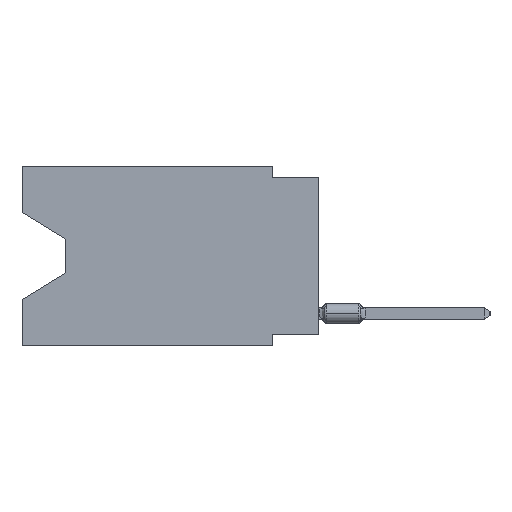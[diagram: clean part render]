
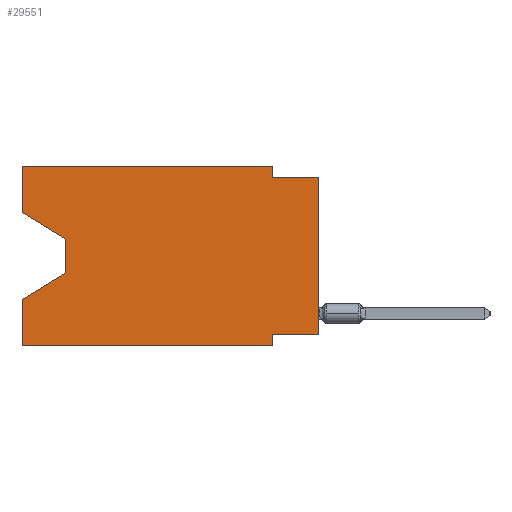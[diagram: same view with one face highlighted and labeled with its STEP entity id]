
A CAD part, left-side view. The second image highlights one B-rep face of the part: STEP entity #29551.
In plain terms, the highlighted planar face has unit normal (-1, 0, 0).
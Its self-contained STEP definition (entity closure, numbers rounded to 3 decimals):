
#448 = LINE ( 'NONE', #6005, #9461 ) ;
#679 = LINE ( 'NONE', #26316, #11996 ) ;
#775 = CARTESIAN_POINT ( 'NONE',  ( 0., 2.54, 0. ) ) ;
#1828 = VECTOR ( 'NONE', #32775, 1000. ) ;
#2061 = VERTEX_POINT ( 'NONE', #11867 ) ;
#2332 = ORIENTED_EDGE ( 'NONE', *, *, #27946, .T. ) ;
#2403 = AXIS2_PLACEMENT_3D ( 'NONE', #29248, #6154, #24351 ) ;
#2508 = CARTESIAN_POINT ( 'NONE',  ( 0., 0., -0.635 ) ) ;
#2751 = EDGE_CURVE ( 'NONE', #22039, #10640, #679, .T. ) ;
#3446 = CARTESIAN_POINT ( 'NONE',  ( 0., 13.97, -5.893 ) ) ;
#3565 = CARTESIAN_POINT ( 'NONE',  ( 0., 2.54, -0.635 ) ) ;
#3770 = LINE ( 'NONE', #4267, #6406 ) ;
#4206 = ORIENTED_EDGE ( 'NONE', *, *, #32711, .F. ) ;
#4267 = CARTESIAN_POINT ( 'NONE',  ( 0., 0., 0. ) ) ;
#4527 = VECTOR ( 'NONE', #31178, 1000. ) ;
#4902 = EDGE_CURVE ( 'NONE', #11299, #10640, #3770, .T. ) ;
#5453 = DIRECTION ( 'NONE',  ( 0., 1., 0. ) ) ;
#5502 = DIRECTION ( 'NONE',  ( 0., -0.855, -0.519 ) ) ;
#5620 = LINE ( 'NONE', #18114, #32018 ) ;
#5708 = DIRECTION ( 'NONE',  ( 0., -1., 0. ) ) ;
#5811 = VERTEX_POINT ( 'NONE', #30617 ) ;
#5850 = CARTESIAN_POINT ( 'NONE',  ( 0., 16.383, -7.36 ) ) ;
#6005 = CARTESIAN_POINT ( 'NONE',  ( 0., 16.383, -2.546 ) ) ;
#6154 = DIRECTION ( 'NONE',  ( 1., 0., 0. ) ) ;
#6406 = VECTOR ( 'NONE', #21792, 1000. ) ;
#7443 = LINE ( 'NONE', #9958, #22364 ) ;
#7466 = EDGE_CURVE ( 'NONE', #18570, #10841, #23406, .T. ) ;
#7983 = EDGE_CURVE ( 'NONE', #12287, #2061, #448, .T. ) ;
#8446 = DIRECTION ( 'NONE',  ( 0., -1., 0. ) ) ;
#8540 = EDGE_CURVE ( 'NONE', #11299, #9713, #5620, .T. ) ;
#8933 = LINE ( 'NONE', #24431, #16962 ) ;
#8987 = VERTEX_POINT ( 'NONE', #775 ) ;
#9274 = VERTEX_POINT ( 'NONE', #27736 ) ;
#9461 = VECTOR ( 'NONE', #5502, 1000. ) ;
#9598 = DIRECTION ( 'NONE',  ( 0., 0., -1. ) ) ;
#9713 = VERTEX_POINT ( 'NONE', #28041 ) ;
#9806 = EDGE_CURVE ( 'NONE', #8987, #22039, #18074, .T. ) ;
#9958 = CARTESIAN_POINT ( 'NONE',  ( 0., 2.54, -9.906 ) ) ;
#10609 = CARTESIAN_POINT ( 'NONE',  ( 0., 16.383, 0. ) ) ;
#10640 = VERTEX_POINT ( 'NONE', #2508 ) ;
#10841 = VERTEX_POINT ( 'NONE', #5850 ) ;
#11116 = ORIENTED_EDGE ( 'NONE', *, *, #14763, .F. ) ;
#11299 = VERTEX_POINT ( 'NONE', #20805 ) ;
#11867 = CARTESIAN_POINT ( 'NONE',  ( 0., 13.97, -4.013 ) ) ;
#11996 = VECTOR ( 'NONE', #8446, 1000. ) ;
#12287 = VERTEX_POINT ( 'NONE', #14750 ) ;
#12697 = CARTESIAN_POINT ( 'NONE',  ( 0., 16.383, -9.906 ) ) ;
#13903 = PLANE ( 'NONE',  #2403 ) ;
#14079 = EDGE_CURVE ( 'NONE', #18570, #9274, #14881, .T. ) ;
#14750 = CARTESIAN_POINT ( 'NONE',  ( 0., 16.383, -2.546 ) ) ;
#14763 = EDGE_CURVE ( 'NONE', #5811, #8987, #23402, .T. ) ;
#14881 = LINE ( 'NONE', #12697, #1828 ) ;
#15157 = ORIENTED_EDGE ( 'NONE', *, *, #31371, .F. ) ;
#15561 = VECTOR ( 'NONE', #16416, 1000. ) ;
#16416 = DIRECTION ( 'NONE',  ( 0., 0.855, -0.519 ) ) ;
#16758 = FACE_OUTER_BOUND ( 'NONE', #26037, .T. ) ;
#16962 = VECTOR ( 'NONE', #32370, 1000. ) ;
#17467 = VECTOR ( 'NONE', #5708, 1000. ) ;
#18067 = ORIENTED_EDGE ( 'NONE', *, *, #8540, .F. ) ;
#18074 = LINE ( 'NONE', #20750, #31815 ) ;
#18114 = CARTESIAN_POINT ( 'NONE',  ( 0., 0., -9.271 ) ) ;
#18570 = VERTEX_POINT ( 'NONE', #31548 ) ;
#19299 = VERTEX_POINT ( 'NONE', #25590 ) ;
#20232 = DIRECTION ( 'NONE',  ( 0., 0., -1. ) ) ;
#20750 = CARTESIAN_POINT ( 'NONE',  ( 0., 2.54, 0. ) ) ;
#20805 = CARTESIAN_POINT ( 'NONE',  ( 0., 0., -9.271 ) ) ;
#21792 = DIRECTION ( 'NONE',  ( 0., 0., 1. ) ) ;
#22039 = VERTEX_POINT ( 'NONE', #3565 ) ;
#22364 = VECTOR ( 'NONE', #20232, 1000. ) ;
#23360 = EDGE_CURVE ( 'NONE', #2061, #19299, #29831, .T. ) ;
#23402 = LINE ( 'NONE', #28488, #17467 ) ;
#23406 = LINE ( 'NONE', #10609, #4527 ) ;
#24175 = LINE ( 'NONE', #3446, #15561 ) ;
#24351 = DIRECTION ( 'NONE',  ( 0., 0., -1. ) ) ;
#24431 = CARTESIAN_POINT ( 'NONE',  ( 0., 16.383, 0. ) ) ;
#25177 = ORIENTED_EDGE ( 'NONE', *, *, #23360, .T. ) ;
#25590 = CARTESIAN_POINT ( 'NONE',  ( 0., 13.97, -5.893 ) ) ;
#26037 = EDGE_LOOP ( 'NONE', ( #33120, #25177, #2332, #32215, #29754, #15157, #18067, #31595, #32253, #33312, #11116, #4206 ) ) ;
#26316 = CARTESIAN_POINT ( 'NONE',  ( 0., 0., -0.635 ) ) ;
#27736 = CARTESIAN_POINT ( 'NONE',  ( 0., 2.54, -9.906 ) ) ;
#27926 = VECTOR ( 'NONE', #9598, 1000. ) ;
#27946 = EDGE_CURVE ( 'NONE', #19299, #10841, #24175, .T. ) ;
#28041 = CARTESIAN_POINT ( 'NONE',  ( 0., 2.54, -9.271 ) ) ;
#28488 = CARTESIAN_POINT ( 'NONE',  ( 0., 16.383, 0. ) ) ;
#28690 = DIRECTION ( 'NONE',  ( 0., 0., -1. ) ) ;
#29248 = CARTESIAN_POINT ( 'NONE',  ( 0., 16.383, 0. ) ) ;
#29551 = ADVANCED_FACE ( 'NONE', ( #16758 ), #13903, .F. ) ;
#29754 = ORIENTED_EDGE ( 'NONE', *, *, #14079, .T. ) ;
#29831 = LINE ( 'NONE', #32718, #27926 ) ;
#30617 = CARTESIAN_POINT ( 'NONE',  ( 0., 16.383, 0. ) ) ;
#31178 = DIRECTION ( 'NONE',  ( 0., 0., 1. ) ) ;
#31371 = EDGE_CURVE ( 'NONE', #9713, #9274, #7443, .T. ) ;
#31548 = CARTESIAN_POINT ( 'NONE',  ( 0., 16.383, -9.906 ) ) ;
#31595 = ORIENTED_EDGE ( 'NONE', *, *, #4902, .T. ) ;
#31815 = VECTOR ( 'NONE', #28690, 1000. ) ;
#32018 = VECTOR ( 'NONE', #5453, 1000. ) ;
#32215 = ORIENTED_EDGE ( 'NONE', *, *, #7466, .F. ) ;
#32253 = ORIENTED_EDGE ( 'NONE', *, *, #2751, .F. ) ;
#32370 = DIRECTION ( 'NONE',  ( 0., 0., 1. ) ) ;
#32711 = EDGE_CURVE ( 'NONE', #12287, #5811, #8933, .T. ) ;
#32718 = CARTESIAN_POINT ( 'NONE',  ( 0., 13.97, -4.013 ) ) ;
#32775 = DIRECTION ( 'NONE',  ( 0., -1., 0. ) ) ;
#33120 = ORIENTED_EDGE ( 'NONE', *, *, #7983, .T. ) ;
#33312 = ORIENTED_EDGE ( 'NONE', *, *, #9806, .F. ) ;
